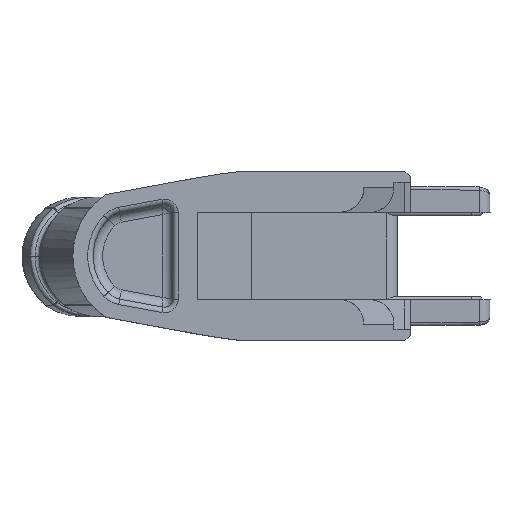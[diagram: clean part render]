
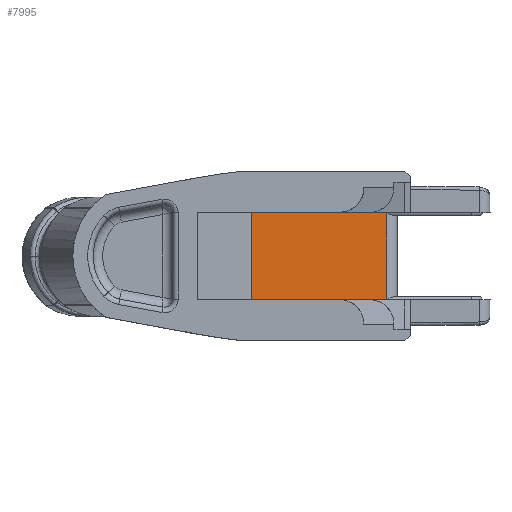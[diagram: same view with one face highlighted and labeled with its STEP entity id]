
A CAD part, top view. The second image highlights one B-rep face of the part: STEP entity #7995.
In plain terms, the highlighted planar face has unit normal (0.002, 0, 1).
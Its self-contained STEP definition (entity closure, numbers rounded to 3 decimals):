
#861=PLANE('',#8635);
#1074=LINE('',#18361,#1438);
#1095=LINE('',#20568,#1459);
#1096=LINE('',#20578,#1460);
#1097=LINE('',#20580,#1461);
#1098=LINE('',#20582,#1462);
#1099=LINE('',#20584,#1463);
#1100=LINE('',#20585,#1464);
#1101=LINE('',#20586,#1465);
#1438=VECTOR('',#9757,10.);
#1459=VECTOR('',#9856,10.);
#1460=VECTOR('',#9859,10.);
#1461=VECTOR('',#9860,10.);
#1462=VECTOR('',#9861,10.);
#1463=VECTOR('',#9862,10.);
#1464=VECTOR('',#9863,10.);
#1465=VECTOR('',#9864,10.);
#2067=FACE_OUTER_BOUND('',#2582,.T.);
#2582=EDGE_LOOP('',(#6580,#6581,#6582,#6583,#6584,#6585,#6586,#6587));
#3548=VERTEX_POINT('',#18357);
#3549=VERTEX_POINT('',#18359);
#3625=VERTEX_POINT('',#20567);
#3626=VERTEX_POINT('',#20576);
#3627=VERTEX_POINT('',#20577);
#3628=VERTEX_POINT('',#20579);
#3629=VERTEX_POINT('',#20581);
#3630=VERTEX_POINT('',#20583);
#4541=EDGE_CURVE('',#3548,#3549,#1074,.T.);
#4669=EDGE_CURVE('',#3548,#3625,#1095,.T.);
#4671=EDGE_CURVE('',#3626,#3627,#1096,.T.);
#4672=EDGE_CURVE('',#3628,#3627,#1097,.T.);
#4673=EDGE_CURVE('',#3629,#3628,#1098,.T.);
#4674=EDGE_CURVE('',#3630,#3629,#1099,.T.);
#4675=EDGE_CURVE('',#3630,#3625,#1100,.T.);
#4676=EDGE_CURVE('',#3549,#3626,#1101,.T.);
#6580=ORIENTED_EDGE('',*,*,#4671,.T.);
#6581=ORIENTED_EDGE('',*,*,#4672,.F.);
#6582=ORIENTED_EDGE('',*,*,#4673,.F.);
#6583=ORIENTED_EDGE('',*,*,#4674,.F.);
#6584=ORIENTED_EDGE('',*,*,#4675,.T.);
#6585=ORIENTED_EDGE('',*,*,#4669,.F.);
#6586=ORIENTED_EDGE('',*,*,#4541,.T.);
#6587=ORIENTED_EDGE('',*,*,#4676,.T.);
#7995=ADVANCED_FACE('',(#2067),#861,.T.);
#8635=AXIS2_PLACEMENT_3D('',#20575,#9857,#9858);
#9757=DIRECTION('',(0.,1.,0.));
#9856=DIRECTION('',(-1.,0.,0.002));
#9857=DIRECTION('center_axis',(0.002,0.,
1.));
#9858=DIRECTION('ref_axis',(1.,0.,-0.002));
#9859=DIRECTION('',(0.,-1.,0.));
#9860=DIRECTION('',(-1.,0.,0.002));
#9861=DIRECTION('',(0.,-1.,0.));
#9862=DIRECTION('',(1.,0.,-0.002));
#9863=DIRECTION('',(0.,1.,0.));
#9864=DIRECTION('',(-1.,0.,0.002));
#18357=CARTESIAN_POINT('',(-123.958,23.19,-27.646));
#18359=CARTESIAN_POINT('',(-123.958,23.24,-27.646));
#18361=CARTESIAN_POINT('',(-123.958,24.701,-27.646));
#20567=CARTESIAN_POINT('',(-139.416,23.19,-27.619));
#20568=CARTESIAN_POINT('',(-124.727,23.19,-27.645));
#20575=CARTESIAN_POINT('Origin',(-139.161,7.24,-27.619));
#20576=CARTESIAN_POINT('',(-174.166,23.24,-27.556));
#20577=CARTESIAN_POINT('',(-174.166,7.24,-27.556));
#20578=CARTESIAN_POINT('',(-174.166,23.24,-27.556));
#20579=CARTESIAN_POINT('',(-123.958,7.24,-27.646));
#20580=CARTESIAN_POINT('',(-143.664,7.24,-27.611));
#20581=CARTESIAN_POINT('',(-123.958,7.29,-27.646));
#20582=CARTESIAN_POINT('',(-123.958,5.779,-27.646));
#20583=CARTESIAN_POINT('',(-139.416,7.29,-27.619));
#20584=CARTESIAN_POINT('',(-124.727,7.29,-27.645));
#20585=CARTESIAN_POINT('',(-139.416,22.965,-27.619));
#20586=CARTESIAN_POINT('',(-143.664,23.24,-27.611));
